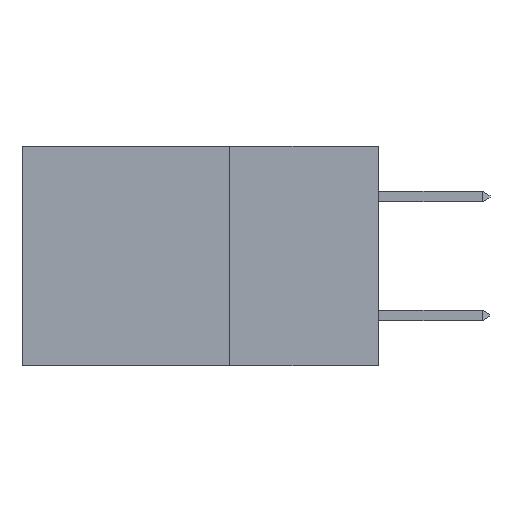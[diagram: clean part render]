
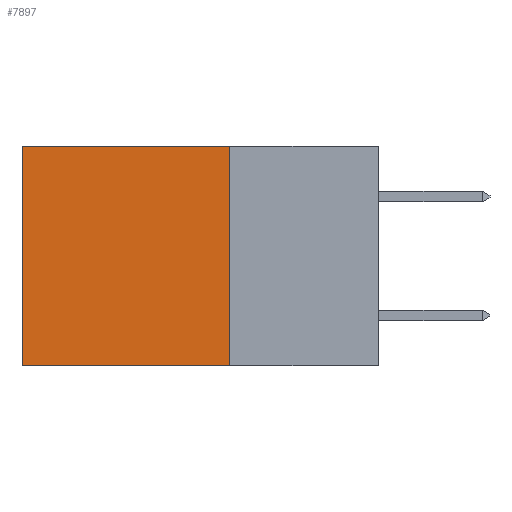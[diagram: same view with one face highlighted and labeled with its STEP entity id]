
A CAD part, left-side view. The second image highlights one B-rep face of the part: STEP entity #7897.
In plain terms, the highlighted planar face has unit normal (-1, 0, 0).
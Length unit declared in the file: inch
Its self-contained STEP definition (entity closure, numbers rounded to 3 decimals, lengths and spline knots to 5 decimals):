
#470 = DIRECTION ( 'NONE',  ( 0., 0., -1. ) ) ;
#480 = PLANE ( 'NONE',  #4294 ) ;
#512 = DIRECTION ( 'NONE',  ( 0., 0., -1. ) ) ;
#736 = ORIENTED_EDGE ( 'NONE', *, *, #9909, .F. ) ;
#745 = CARTESIAN_POINT ( 'NONE',  ( 0.298, 0.25, 0. ) ) ;
#1605 = DIRECTION ( 'NONE',  ( 0., 1., 0. ) ) ;
#2179 = CARTESIAN_POINT ( 'NONE',  ( 0.298, 0.25, 0. ) ) ;
#2581 = VECTOR ( 'NONE', #7072, 39.37008 ) ;
#2709 = ORIENTED_EDGE ( 'NONE', *, *, #5407, .T. ) ;
#2718 = EDGE_CURVE ( 'NONE', #7922, #4879, #4777, .T. ) ;
#2941 = FACE_OUTER_BOUND ( 'NONE', #7073, .T. ) ;
#2997 = CARTESIAN_POINT ( 'NONE',  ( 0.298, 0.25, 0. ) ) ;
#3001 = VECTOR ( 'NONE', #1605, 39.37008 ) ;
#3038 = DIRECTION ( 'NONE',  ( 0., 0., -1. ) ) ;
#3672 = CARTESIAN_POINT ( 'NONE',  ( 0.298, 0.25, -0.37 ) ) ;
#4294 = AXIS2_PLACEMENT_3D ( 'NONE', #2997, #5482, #512 ) ;
#4556 = CARTESIAN_POINT ( 'NONE',  ( 0.298, 0.6, 0. ) ) ;
#4698 = CARTESIAN_POINT ( 'NONE',  ( 0.298, 0.25, -0.37 ) ) ;
#4777 = LINE ( 'NONE', #3672, #2581 ) ;
#4832 = VERTEX_POINT ( 'NONE', #8987 ) ;
#4879 = VERTEX_POINT ( 'NONE', #6556 ) ;
#5199 = LINE ( 'NONE', #745, #3001 ) ;
#5407 = EDGE_CURVE ( 'NONE', #7809, #4879, #7149, .T. ) ;
#5482 = DIRECTION ( 'NONE',  ( 1., 0., 0. ) ) ;
#6556 = CARTESIAN_POINT ( 'NONE',  ( 0.298, 0.6, -0.37 ) ) ;
#6879 = VECTOR ( 'NONE', #470, 39.37008 ) ;
#7072 = DIRECTION ( 'NONE',  ( 0., 1., 0. ) ) ;
#7073 = EDGE_LOOP ( 'NONE', ( #2709, #9275, #736, #9519 ) ) ;
#7149 = LINE ( 'NONE', #9521, #6879 ) ;
#7291 = EDGE_CURVE ( 'NONE', #4832, #7809, #5199, .T. ) ;
#7667 = VECTOR ( 'NONE', #3038, 39.37008 ) ;
#7809 = VERTEX_POINT ( 'NONE', #4556 ) ;
#7897 = ADVANCED_FACE ( 'NONE', ( #2941 ), #480, .F. ) ;
#7922 = VERTEX_POINT ( 'NONE', #4698 ) ;
#8987 = CARTESIAN_POINT ( 'NONE',  ( 0.298, 0.25, 0. ) ) ;
#9275 = ORIENTED_EDGE ( 'NONE', *, *, #2718, .F. ) ;
#9519 = ORIENTED_EDGE ( 'NONE', *, *, #7291, .T. ) ;
#9521 = CARTESIAN_POINT ( 'NONE',  ( 0.298, 0.6, 0. ) ) ;
#9839 = LINE ( 'NONE', #2179, #7667 ) ;
#9909 = EDGE_CURVE ( 'NONE', #4832, #7922, #9839, .T. ) ;
